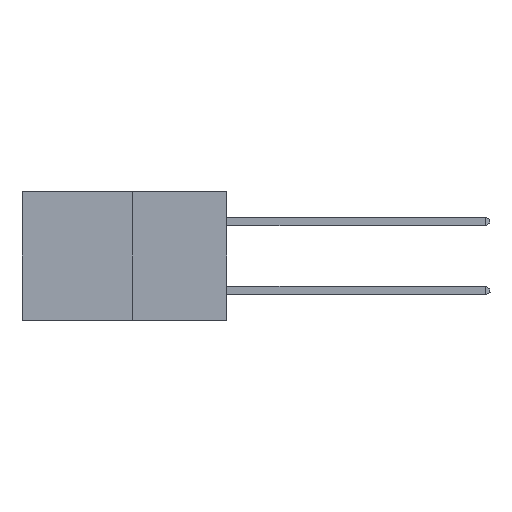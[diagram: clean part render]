
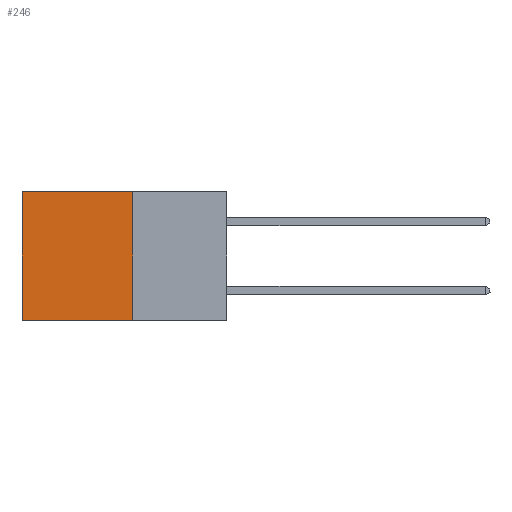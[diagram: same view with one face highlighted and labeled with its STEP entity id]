
A CAD part, left-side view. The second image highlights one B-rep face of the part: STEP entity #246.
In plain terms, the highlighted planar face has unit normal (-1, 0, 0).
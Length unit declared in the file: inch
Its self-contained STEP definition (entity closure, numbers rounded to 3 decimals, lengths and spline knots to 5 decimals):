
#246 = ADVANCED_FACE ( 'NONE', ( #5521 ), #9077, .F. ) ;
#432 = DIRECTION ( 'NONE',  ( 0., 0., -1. ) ) ;
#1111 = CARTESIAN_POINT ( 'NONE',  ( 0.277, 0.27, -0.37 ) ) ;
#1223 = CARTESIAN_POINT ( 'NONE',  ( 0.277, 0.27, -0.37 ) ) ;
#1379 = DIRECTION ( 'NONE',  ( 0., 1., 0. ) ) ;
#1557 = CARTESIAN_POINT ( 'NONE',  ( 0.277, 0.59, -0.37 ) ) ;
#2138 = EDGE_CURVE ( 'NONE', #2164, #4961, #3070, .T. ) ;
#2164 = VERTEX_POINT ( 'NONE', #5913 ) ;
#2175 = VERTEX_POINT ( 'NONE', #3509 ) ;
#2272 = VECTOR ( 'NONE', #10102, 39.37008 ) ;
#2396 = VERTEX_POINT ( 'NONE', #1111 ) ;
#3070 = LINE ( 'NONE', #8747, #7220 ) ;
#3077 = EDGE_CURVE ( 'NONE', #2164, #2396, #4266, .T. ) ;
#3246 = EDGE_CURVE ( 'NONE', #2396, #2175, #8270, .T. ) ;
#3509 = CARTESIAN_POINT ( 'NONE',  ( 0.277, 0.59, -0.37 ) ) ;
#3626 = EDGE_CURVE ( 'NONE', #4961, #2175, #6926, .T. ) ;
#3886 = EDGE_LOOP ( 'NONE', ( #6253, #6326, #6427, #9897 ) ) ;
#3916 = VECTOR ( 'NONE', #1379, 39.37008 ) ;
#4266 = LINE ( 'NONE', #4315, #10142 ) ;
#4315 = CARTESIAN_POINT ( 'NONE',  ( 0.277, 0.27, -0.37 ) ) ;
#4775 = CARTESIAN_POINT ( 'NONE',  ( 0.277, 0.27, -0.37 ) ) ;
#4961 = VERTEX_POINT ( 'NONE', #9578 ) ;
#5447 = DIRECTION ( 'NONE',  ( 0., 0., -1. ) ) ;
#5521 = FACE_OUTER_BOUND ( 'NONE', #3886, .T. ) ;
#5913 = CARTESIAN_POINT ( 'NONE',  ( 0.277, 0.27, 0. ) ) ;
#6253 = ORIENTED_EDGE ( 'NONE', *, *, #3626, .T. ) ;
#6326 = ORIENTED_EDGE ( 'NONE', *, *, #3246, .F. ) ;
#6427 = ORIENTED_EDGE ( 'NONE', *, *, #3077, .F. ) ;
#6437 = AXIS2_PLACEMENT_3D ( 'NONE', #4775, #8730, #5447 ) ;
#6926 = LINE ( 'NONE', #1557, #2272 ) ;
#7220 = VECTOR ( 'NONE', #8278, 39.37008 ) ;
#8270 = LINE ( 'NONE', #1223, #3916 ) ;
#8278 = DIRECTION ( 'NONE',  ( 0., 1., 0. ) ) ;
#8730 = DIRECTION ( 'NONE',  ( 1., 0., 0. ) ) ;
#8747 = CARTESIAN_POINT ( 'NONE',  ( 0.277, 0.27, 0. ) ) ;
#9077 = PLANE ( 'NONE',  #6437 ) ;
#9578 = CARTESIAN_POINT ( 'NONE',  ( 0.277, 0.59, 0. ) ) ;
#9897 = ORIENTED_EDGE ( 'NONE', *, *, #2138, .T. ) ;
#10102 = DIRECTION ( 'NONE',  ( 0., 0., -1. ) ) ;
#10142 = VECTOR ( 'NONE', #432, 39.37008 ) ;
